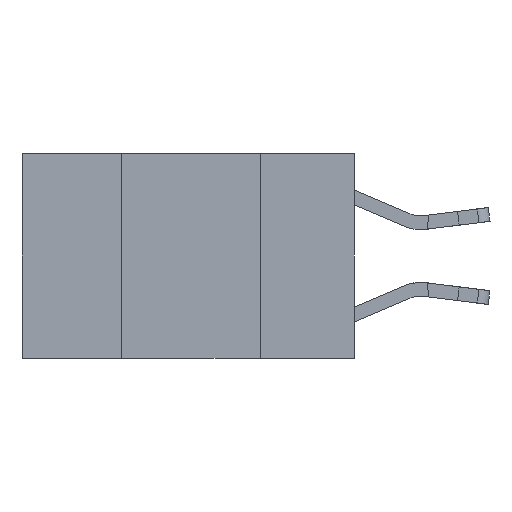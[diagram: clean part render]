
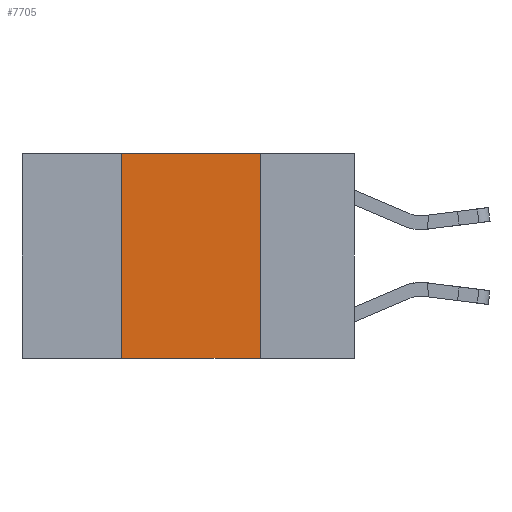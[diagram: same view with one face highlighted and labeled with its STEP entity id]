
A CAD part, left-side view. The second image highlights one B-rep face of the part: STEP entity #7705.
In plain terms, the highlighted planar face has unit normal (-1, 0, 0).
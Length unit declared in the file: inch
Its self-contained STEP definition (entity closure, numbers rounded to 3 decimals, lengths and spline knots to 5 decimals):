
#3 = CARTESIAN_POINT ( 'NONE',  ( 0., 0.42, 0. ) ) ;
#524 = VECTOR ( 'NONE', #1553, 39.37008 ) ;
#565 = CARTESIAN_POINT ( 'NONE',  ( 0., 0.6, 0. ) ) ;
#607 = EDGE_CURVE ( 'NONE', #15513, #3504, #6623, .T. ) ;
#774 = FACE_OUTER_BOUND ( 'NONE', #5916, .T. ) ;
#1448 = ORIENTED_EDGE ( 'NONE', *, *, #9362, .T. ) ;
#1553 = DIRECTION ( 'NONE',  ( 0., 0., -1. ) ) ;
#1800 = CARTESIAN_POINT ( 'NONE',  ( 0., 0.17, -0.37 ) ) ;
#2083 = LINE ( 'NONE', #565, #3733 ) ;
#2489 = LINE ( 'NONE', #3, #8878 ) ;
#3298 = DIRECTION ( 'NONE',  ( 0., -1., 0. ) ) ;
#3348 = PLANE ( 'NONE',  #6377 ) ;
#3504 = VERTEX_POINT ( 'NONE', #1800 ) ;
#3733 = VECTOR ( 'NONE', #3298, 39.37008 ) ;
#4175 = CARTESIAN_POINT ( 'NONE',  ( 0., 0.17, 0. ) ) ;
#4494 = VECTOR ( 'NONE', #16687, 39.37008 ) ;
#5434 = VERTEX_POINT ( 'NONE', #7078 ) ;
#5916 = EDGE_LOOP ( 'NONE', ( #11334, #9349, #9806, #1448 ) ) ;
#6134 = LINE ( 'NONE', #11412, #4494 ) ;
#6377 = AXIS2_PLACEMENT_3D ( 'NONE', #9973, #16635, #15349 ) ;
#6623 = LINE ( 'NONE', #13390, #524 ) ;
#6710 = VERTEX_POINT ( 'NONE', #8919 ) ;
#7078 = CARTESIAN_POINT ( 'NONE',  ( 0., 0.42, -0.37 ) ) ;
#7705 = ADVANCED_FACE ( 'NONE', ( #774 ), #3348, .F. ) ;
#8328 = EDGE_CURVE ( 'NONE', #5434, #6710, #2489, .T. ) ;
#8842 = DIRECTION ( 'NONE',  ( 0., 0., 1. ) ) ;
#8878 = VECTOR ( 'NONE', #8842, 39.37008 ) ;
#8919 = CARTESIAN_POINT ( 'NONE',  ( 0., 0.42, 0. ) ) ;
#9349 = ORIENTED_EDGE ( 'NONE', *, *, #10864, .F. ) ;
#9362 = EDGE_CURVE ( 'NONE', #5434, #3504, #6134, .T. ) ;
#9806 = ORIENTED_EDGE ( 'NONE', *, *, #8328, .F. ) ;
#9973 = CARTESIAN_POINT ( 'NONE',  ( 0., 0.6, 0. ) ) ;
#10864 = EDGE_CURVE ( 'NONE', #6710, #15513, #2083, .T. ) ;
#11334 = ORIENTED_EDGE ( 'NONE', *, *, #607, .F. ) ;
#11412 = CARTESIAN_POINT ( 'NONE',  ( 0., 0.6, -0.37 ) ) ;
#13390 = CARTESIAN_POINT ( 'NONE',  ( 0., 0.17, 0. ) ) ;
#15349 = DIRECTION ( 'NONE',  ( 0., 0., -1. ) ) ;
#15513 = VERTEX_POINT ( 'NONE', #4175 ) ;
#16635 = DIRECTION ( 'NONE',  ( 1., 0., 0. ) ) ;
#16687 = DIRECTION ( 'NONE',  ( 0., -1., 0. ) ) ;
